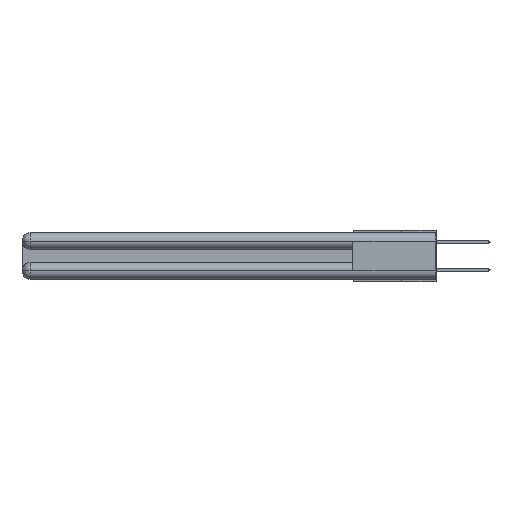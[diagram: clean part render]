
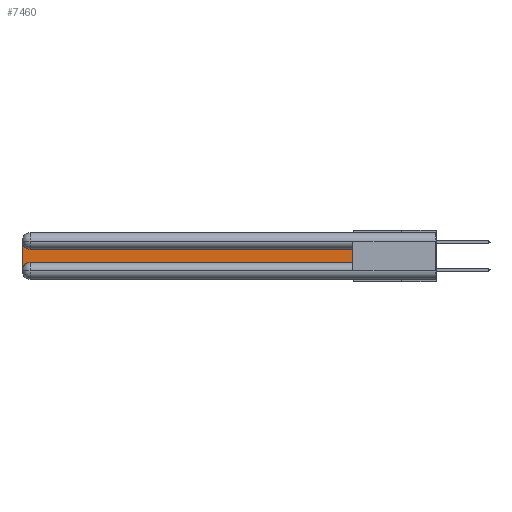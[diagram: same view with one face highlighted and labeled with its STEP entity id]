
A CAD part, left-side view. The second image highlights one B-rep face of the part: STEP entity #7460.
In plain terms, the highlighted planar face has unit normal (-1, 0, 0).
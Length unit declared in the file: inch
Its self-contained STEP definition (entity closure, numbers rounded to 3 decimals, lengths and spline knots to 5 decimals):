
#66 = EDGE_CURVE ( 'NONE', #28111, #17341, #7301, .T. ) ;
#294 = DIRECTION ( 'NONE',  ( 1., 0., 0. ) ) ;
#1421 = DIRECTION ( 'NONE',  ( 0., -1., 0. ) ) ;
#1804 = DIRECTION ( 'NONE',  ( 1., 0., 0. ) ) ;
#2503 = CARTESIAN_POINT ( 'NONE',  ( 0.075, 0.6, -0.2175 ) ) ;
#2584 = EDGE_CURVE ( 'NONE', #5189, #28111, #8979, .T. ) ;
#3042 = ORIENTED_EDGE ( 'NONE', *, *, #6815, .T. ) ;
#3067 = DIRECTION ( 'NONE',  ( 1., 0., 0. ) ) ;
#3156 = DIRECTION ( 'NONE',  ( 0., 0., -1. ) ) ;
#3539 = VECTOR ( 'NONE', #1421, 39.37008 ) ;
#3848 = ORIENTED_EDGE ( 'NONE', *, *, #5764, .T. ) ;
#4457 = ORIENTED_EDGE ( 'NONE', *, *, #12041, .T. ) ;
#5189 = VERTEX_POINT ( 'NONE', #2503 ) ;
#5764 = EDGE_CURVE ( 'NONE', #17341, #19739, #26838, .T. ) ;
#6147 = VERTEX_POINT ( 'NONE', #23918 ) ;
#6815 = EDGE_CURVE ( 'NONE', #21302, #5189, #9441, .T. ) ;
#7301 = LINE ( 'NONE', #26815, #24385 ) ;
#7460 = ADVANCED_FACE ( 'NONE', ( #23305 ), #23120, .F. ) ;
#8979 = LINE ( 'NONE', #13947, #16237 ) ;
#9406 = EDGE_LOOP ( 'NONE', ( #18013, #3848, #4457, #19919, #3042, #22037 ) ) ;
#9441 = LINE ( 'NONE', #21231, #3539 ) ;
#9753 = CARTESIAN_POINT ( 'NONE',  ( 0.075, 2.94, -0.1225 ) ) ;
#9914 = CARTESIAN_POINT ( 'NONE',  ( 0.075, 3., -0.0625 ) ) ;
#11679 = CARTESIAN_POINT ( 'NONE',  ( 0.075, 3., -0.1225 ) ) ;
#12041 = EDGE_CURVE ( 'NONE', #19739, #6147, #18231, .T. ) ;
#13515 = DIRECTION ( 'NONE',  ( 0., 1., 0. ) ) ;
#13599 = DIRECTION ( 'NONE',  ( 0., 0., -1. ) ) ;
#13896 = EDGE_CURVE ( 'NONE', #6147, #21302, #24930, .T. ) ;
#13947 = CARTESIAN_POINT ( 'NONE',  ( 0.075, 0.6, -0.2175 ) ) ;
#16237 = VECTOR ( 'NONE', #22676, 39.37008 ) ;
#17341 = VERTEX_POINT ( 'NONE', #9753 ) ;
#18013 = ORIENTED_EDGE ( 'NONE', *, *, #66, .T. ) ;
#18231 = LINE ( 'NONE', #18547, #18566 ) ;
#18449 = CARTESIAN_POINT ( 'NONE',  ( 0.075, 2.94, -0.2175 ) ) ;
#18547 = CARTESIAN_POINT ( 'NONE',  ( 0.075, 3., -0.2175 ) ) ;
#18566 = VECTOR ( 'NONE', #25785, 39.37008 ) ;
#19739 = VERTEX_POINT ( 'NONE', #9914 ) ;
#19919 = ORIENTED_EDGE ( 'NONE', *, *, #13896, .T. ) ;
#21231 = CARTESIAN_POINT ( 'NONE',  ( 0.075, 0.6, -0.2175 ) ) ;
#21302 = VERTEX_POINT ( 'NONE', #18449 ) ;
#21951 = AXIS2_PLACEMENT_3D ( 'NONE', #23057, #3067, #3156 ) ;
#22037 = ORIENTED_EDGE ( 'NONE', *, *, #2584, .T. ) ;
#22155 = AXIS2_PLACEMENT_3D ( 'NONE', #11679, #1804, #28621 ) ;
#22527 = CARTESIAN_POINT ( 'NONE',  ( 0.075, 2.94, -0.2775 ) ) ;
#22605 = AXIS2_PLACEMENT_3D ( 'NONE', #22527, #294, #13599 ) ;
#22676 = DIRECTION ( 'NONE',  ( 0., 0., 1. ) ) ;
#23057 = CARTESIAN_POINT ( 'NONE',  ( 0.075, 2.94, -0.0625 ) ) ;
#23120 = PLANE ( 'NONE',  #22155 ) ;
#23305 = FACE_OUTER_BOUND ( 'NONE', #9406, .T. ) ;
#23918 = CARTESIAN_POINT ( 'NONE',  ( 0.075, 3., -0.2775 ) ) ;
#24385 = VECTOR ( 'NONE', #13515, 39.37008 ) ;
#24930 = CIRCLE ( 'NONE', #22605, 0.06 ) ;
#25785 = DIRECTION ( 'NONE',  ( 0., 0., -1. ) ) ;
#26182 = CARTESIAN_POINT ( 'NONE',  ( 0.075, 0.6, -0.1225 ) ) ;
#26815 = CARTESIAN_POINT ( 'NONE',  ( 0.075, 0.6, -0.1225 ) ) ;
#26838 = CIRCLE ( 'NONE', #21951, 0.06 ) ;
#28111 = VERTEX_POINT ( 'NONE', #26182 ) ;
#28621 = DIRECTION ( 'NONE',  ( 0., 0., -1. ) ) ;
